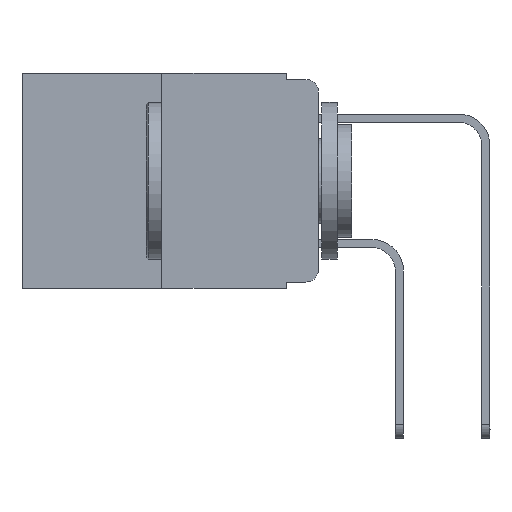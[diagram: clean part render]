
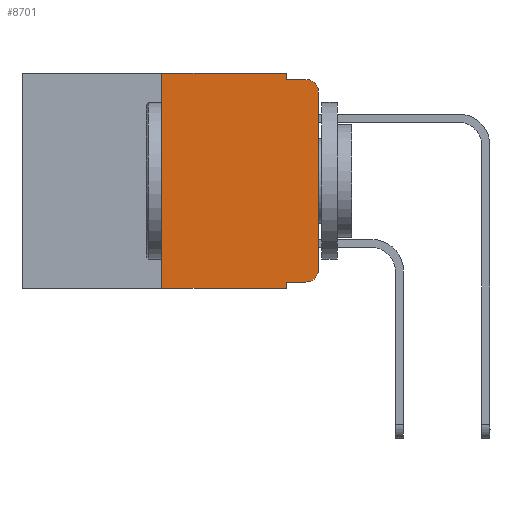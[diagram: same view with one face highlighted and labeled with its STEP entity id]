
A CAD part, left-side view. The second image highlights one B-rep face of the part: STEP entity #8701.
In plain terms, the highlighted planar face has unit normal (-1, 0, 0).
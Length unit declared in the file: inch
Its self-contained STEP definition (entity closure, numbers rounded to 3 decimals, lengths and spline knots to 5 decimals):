
#201 = ORIENTED_EDGE ( 'NONE', *, *, #11423, .F. ) ;
#426 = LINE ( 'NONE', #8676, #11957 ) ;
#1273 = VERTEX_POINT ( 'NONE', #12245 ) ;
#1315 = VERTEX_POINT ( 'NONE', #12415 ) ;
#1368 = VERTEX_POINT ( 'NONE', #6453 ) ;
#1490 = DIRECTION ( 'NONE',  ( 0., 0., 1. ) ) ;
#1512 = CARTESIAN_POINT ( 'NONE',  ( 0., 0., -0.313 ) ) ;
#1542 = AXIS2_PLACEMENT_3D ( 'NONE', #5093, #12151, #3026 ) ;
#1623 = CARTESIAN_POINT ( 'NONE',  ( 0., 0.051, -0.343 ) ) ;
#1768 = CARTESIAN_POINT ( 'NONE',  ( 0., 0.25, 0. ) ) ;
#1849 = CIRCLE ( 'NONE', #10750, 0.02 ) ;
#1875 = EDGE_CURVE ( 'NONE', #1368, #1315, #9393, .T. ) ;
#2043 = DIRECTION ( 'NONE',  ( 0., -1., 0. ) ) ;
#2094 = CARTESIAN_POINT ( 'NONE',  ( 0., 0.051, 0. ) ) ;
#2393 = VECTOR ( 'NONE', #9582, 39.37008 ) ;
#2441 = CARTESIAN_POINT ( 'NONE',  ( 0., 0.02, -0.313 ) ) ;
#2507 = VECTOR ( 'NONE', #2043, 39.37008 ) ;
#2538 = CARTESIAN_POINT ( 'NONE',  ( 0., 0.473, -0.343 ) ) ;
#2577 = ORIENTED_EDGE ( 'NONE', *, *, #8819, .T. ) ;
#3026 = DIRECTION ( 'NONE',  ( 0., 0., -1. ) ) ;
#3059 = CARTESIAN_POINT ( 'NONE',  ( 0., 0.473, 0. ) ) ;
#3170 = VERTEX_POINT ( 'NONE', #8009 ) ;
#3285 = DIRECTION ( 'NONE',  ( 0., -1., 0. ) ) ;
#3594 = ORIENTED_EDGE ( 'NONE', *, *, #9003, .T. ) ;
#3598 = EDGE_CURVE ( 'NONE', #1273, #1315, #8607, .T. ) ;
#3950 = EDGE_CURVE ( 'NONE', #3170, #12027, #6332, .T. ) ;
#3998 = ORIENTED_EDGE ( 'NONE', *, *, #3598, .F. ) ;
#4251 = CARTESIAN_POINT ( 'NONE',  ( 0., 0.051, -0.333 ) ) ;
#4296 = DIRECTION ( 'NONE',  ( 0., 0., -1. ) ) ;
#4522 = DIRECTION ( 'NONE',  ( 0., -1., 0. ) ) ;
#4779 = VERTEX_POINT ( 'NONE', #7055 ) ;
#4791 = VERTEX_POINT ( 'NONE', #11964 ) ;
#5093 = CARTESIAN_POINT ( 'NONE',  ( 0., 0.473, 0. ) ) ;
#5163 = LINE ( 'NONE', #5831, #10815 ) ;
#5190 = FACE_OUTER_BOUND ( 'NONE', #10593, .T. ) ;
#5196 = CARTESIAN_POINT ( 'NONE',  ( 0., 0.02, -0.333 ) ) ;
#5350 = DIRECTION ( 'NONE',  ( -1., 0., 0. ) ) ;
#5389 = EDGE_CURVE ( 'NONE', #9120, #4779, #5813, .T. ) ;
#5669 = EDGE_CURVE ( 'NONE', #3170, #9120, #9447, .T. ) ;
#5810 = EDGE_CURVE ( 'NONE', #7718, #1368, #426, .T. ) ;
#5813 = LINE ( 'NONE', #3059, #2507 ) ;
#5831 = CARTESIAN_POINT ( 'NONE',  ( 0., 0.051, 0. ) ) ;
#6043 = AXIS2_PLACEMENT_3D ( 'NONE', #10359, #5350, #4296 ) ;
#6184 = DIRECTION ( 'NONE',  ( 0., 0., -1. ) ) ;
#6332 = LINE ( 'NONE', #2538, #2393 ) ;
#6432 = ORIENTED_EDGE ( 'NONE', *, *, #5389, .F. ) ;
#6453 = CARTESIAN_POINT ( 'NONE',  ( 0., 0., -0.03 ) ) ;
#6540 = VECTOR ( 'NONE', #4522, 39.37008 ) ;
#6562 = ORIENTED_EDGE ( 'NONE', *, *, #5669, .F. ) ;
#6570 = ORIENTED_EDGE ( 'NONE', *, *, #1875, .T. ) ;
#6706 = DIRECTION ( 'NONE',  ( 0., 0., -1. ) ) ;
#7055 = CARTESIAN_POINT ( 'NONE',  ( 0., 0.051, 0. ) ) ;
#7361 = CARTESIAN_POINT ( 'NONE',  ( 0., 0.25, 0. ) ) ;
#7718 = VERTEX_POINT ( 'NONE', #1512 ) ;
#8009 = CARTESIAN_POINT ( 'NONE',  ( 0., 0.25, -0.343 ) ) ;
#8607 = LINE ( 'NONE', #9628, #6540 ) ;
#8676 = CARTESIAN_POINT ( 'NONE',  ( 0., 0., 0. ) ) ;
#8684 = EDGE_CURVE ( 'NONE', #4779, #1273, #13045, .T. ) ;
#8701 = ADVANCED_FACE ( 'NONE', ( #5190 ), #9055, .F. ) ;
#8738 = ORIENTED_EDGE ( 'NONE', *, *, #3950, .T. ) ;
#8819 = EDGE_CURVE ( 'NONE', #4791, #11139, #9572, .T. ) ;
#9003 = EDGE_CURVE ( 'NONE', #11139, #7718, #1849, .T. ) ;
#9055 = PLANE ( 'NONE',  #1542 ) ;
#9120 = VERTEX_POINT ( 'NONE', #1768 ) ;
#9393 = CIRCLE ( 'NONE', #6043, 0.02 ) ;
#9398 = ORIENTED_EDGE ( 'NONE', *, *, #8684, .F. ) ;
#9447 = LINE ( 'NONE', #7361, #10526 ) ;
#9572 = LINE ( 'NONE', #4251, #11631 ) ;
#9582 = DIRECTION ( 'NONE',  ( 0., -1., 0. ) ) ;
#9628 = CARTESIAN_POINT ( 'NONE',  ( 0., 0.051, -0.01 ) ) ;
#10272 = ORIENTED_EDGE ( 'NONE', *, *, #5810, .T. ) ;
#10359 = CARTESIAN_POINT ( 'NONE',  ( 0., 0.02, -0.03 ) ) ;
#10362 = VECTOR ( 'NONE', #6184, 39.37008 ) ;
#10526 = VECTOR ( 'NONE', #1490, 39.37008 ) ;
#10593 = EDGE_LOOP ( 'NONE', ( #10272, #6570, #3998, #9398, #6432, #6562, #8738, #201, #2577, #3594 ) ) ;
#10750 = AXIS2_PLACEMENT_3D ( 'NONE', #2441, #11594, #11642 ) ;
#10815 = VECTOR ( 'NONE', #6706, 39.37008 ) ;
#11139 = VERTEX_POINT ( 'NONE', #5196 ) ;
#11423 = EDGE_CURVE ( 'NONE', #4791, #12027, #5163, .T. ) ;
#11594 = DIRECTION ( 'NONE',  ( -1., 0., 0. ) ) ;
#11631 = VECTOR ( 'NONE', #3285, 39.37008 ) ;
#11642 = DIRECTION ( 'NONE',  ( 0., 0., -1. ) ) ;
#11957 = VECTOR ( 'NONE', #12727, 39.37008 ) ;
#11964 = CARTESIAN_POINT ( 'NONE',  ( 0., 0.051, -0.333 ) ) ;
#12027 = VERTEX_POINT ( 'NONE', #1623 ) ;
#12151 = DIRECTION ( 'NONE',  ( 1., 0., 0. ) ) ;
#12245 = CARTESIAN_POINT ( 'NONE',  ( 0., 0.051, -0.01 ) ) ;
#12415 = CARTESIAN_POINT ( 'NONE',  ( 0., 0.02, -0.01 ) ) ;
#12727 = DIRECTION ( 'NONE',  ( 0., 0., 1. ) ) ;
#13045 = LINE ( 'NONE', #2094, #10362 ) ;
